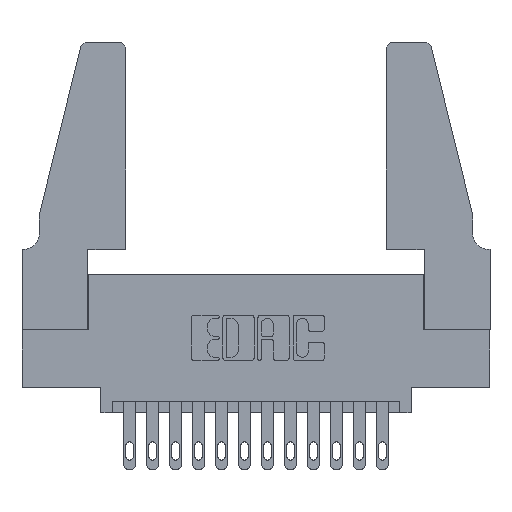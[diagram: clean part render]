
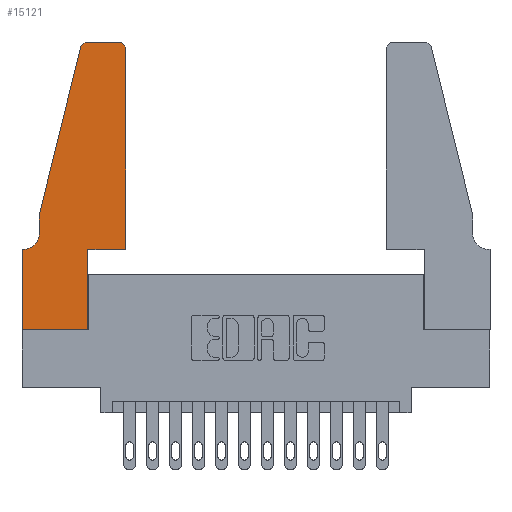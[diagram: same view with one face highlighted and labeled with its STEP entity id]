
A CAD part, top view. The second image highlights one B-rep face of the part: STEP entity #15121.
In plain terms, the highlighted planar face has unit normal (0, 0, 1).
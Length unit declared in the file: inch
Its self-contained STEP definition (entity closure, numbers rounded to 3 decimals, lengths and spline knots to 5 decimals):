
#67 = EDGE_CURVE ( 'NONE', #5300, #13426, #7095, .T. ) ;
#157 = VECTOR ( 'NONE', #8464, 39.37008 ) ;
#318 = LINE ( 'NONE', #5519, #14913 ) ;
#465 = CARTESIAN_POINT ( 'NONE',  ( 0., 0.35, 0.37 ) ) ;
#573 = EDGE_CURVE ( 'NONE', #2200, #4319, #5377, .T. ) ;
#613 = AXIS2_PLACEMENT_3D ( 'NONE', #645, #13891, #11361 ) ;
#630 = VERTEX_POINT ( 'NONE', #9015 ) ;
#645 = CARTESIAN_POINT ( 'NONE',  ( 0.284, 1.22, 0.37 ) ) ;
#835 = ORIENTED_EDGE ( 'NONE', *, *, #67, .T. ) ;
#865 = FACE_OUTER_BOUND ( 'NONE', #1805, .T. ) ;
#1190 = LINE ( 'NONE', #7786, #9736 ) ;
#1316 = EDGE_CURVE ( 'NONE', #12863, #2200, #9696, .T. ) ;
#1805 = EDGE_LOOP ( 'NONE', ( #11169, #7963, #5261, #4058, #13999, #9672, #11109, #8523, #835, #10504, #7614, #3324 ) ) ;
#1875 = DIRECTION ( 'NONE',  ( 0., -1., 0. ) ) ;
#1918 = EDGE_CURVE ( 'NONE', #13426, #11104, #13650, .T. ) ;
#2200 = VERTEX_POINT ( 'NONE', #2621 ) ;
#2281 = VECTOR ( 'NONE', #5505, 39.37008 ) ;
#2303 = EDGE_CURVE ( 'NONE', #630, #12023, #2631, .T. ) ;
#2348 = DIRECTION ( 'NONE',  ( 1., 0., 0. ) ) ;
#2621 = CARTESIAN_POINT ( 'NONE',  ( 0.284, 1.25, 0.37 ) ) ;
#2626 = AXIS2_PLACEMENT_3D ( 'NONE', #8407, #15666, #2348 ) ;
#2631 = CIRCLE ( 'NONE', #3877, 0.07 ) ;
#2777 = VECTOR ( 'NONE', #5715, 39.37008 ) ;
#3317 = DIRECTION ( 'NONE',  ( 0., 0., -1. ) ) ;
#3324 = ORIENTED_EDGE ( 'NONE', *, *, #9983, .T. ) ;
#3445 = EDGE_CURVE ( 'NONE', #5914, #4510, #318, .T. ) ;
#3466 = VECTOR ( 'NONE', #14533, 39.37008 ) ;
#3470 = EDGE_CURVE ( 'NONE', #13828, #630, #10181, .T. ) ;
#3681 = CARTESIAN_POINT ( 'NONE',  ( 0.0755, 0.35, 0.37 ) ) ;
#3877 = AXIS2_PLACEMENT_3D ( 'NONE', #9301, #3317, #5675 ) ;
#3904 = CARTESIAN_POINT ( 'NONE',  ( 0.4205, 1.25, 0.37 ) ) ;
#4052 = LINE ( 'NONE', #4678, #10135 ) ;
#4058 = ORIENTED_EDGE ( 'NONE', *, *, #3470, .T. ) ;
#4319 = VERTEX_POINT ( 'NONE', #11780 ) ;
#4510 = VERTEX_POINT ( 'NONE', #10077 ) ;
#4678 = CARTESIAN_POINT ( 'NONE',  ( 0., 0., 0.37 ) ) ;
#4879 = PLANE ( 'NONE',  #13546 ) ;
#5085 = DIRECTION ( 'NONE',  ( 1., 0., 0. ) ) ;
#5261 = ORIENTED_EDGE ( 'NONE', *, *, #14078, .T. ) ;
#5300 = VERTEX_POINT ( 'NONE', #12342 ) ;
#5377 = CIRCLE ( 'NONE', #613, 0.03 ) ;
#5505 = DIRECTION ( 'NONE',  ( -1., 0., 0. ) ) ;
#5519 = CARTESIAN_POINT ( 'NONE',  ( 0., 0., 0.37 ) ) ;
#5675 = DIRECTION ( 'NONE',  ( -1., 0., 0. ) ) ;
#5715 = DIRECTION ( 'NONE',  ( -0.239, -0.971, 0. ) ) ;
#5914 = VERTEX_POINT ( 'NONE', #465 ) ;
#6298 = CARTESIAN_POINT ( 'NONE',  ( 0., 0.35, 0.37 ) ) ;
#6673 = EDGE_CURVE ( 'NONE', #11104, #7295, #1190, .T. ) ;
#7095 = LINE ( 'NONE', #8273, #3466 ) ;
#7295 = VERTEX_POINT ( 'NONE', #11320 ) ;
#7614 = ORIENTED_EDGE ( 'NONE', *, *, #6673, .T. ) ;
#7770 = CARTESIAN_POINT ( 'NONE',  ( 0.0755, 0.5, 0.37 ) ) ;
#7786 = CARTESIAN_POINT ( 'NONE',  ( 0.4505, 0.35, 0.37 ) ) ;
#7926 = LINE ( 'NONE', #3681, #157 ) ;
#7963 = ORIENTED_EDGE ( 'NONE', *, *, #573, .T. ) ;
#7982 = CARTESIAN_POINT ( 'NONE',  ( 0.0755, 0.5, 0.37 ) ) ;
#8248 = DIRECTION ( 'NONE',  ( 1., 0., 0. ) ) ;
#8273 = CARTESIAN_POINT ( 'NONE',  ( 0.2865, 0.35, 0.37 ) ) ;
#8407 = CARTESIAN_POINT ( 'NONE',  ( 0.4205, 1.22, 0.37 ) ) ;
#8439 = DIRECTION ( 'NONE',  ( 0., 0., 1. ) ) ;
#8464 = DIRECTION ( 'NONE',  ( -1., 0., 0. ) ) ;
#8523 = ORIENTED_EDGE ( 'NONE', *, *, #10004, .T. ) ;
#8655 = CARTESIAN_POINT ( 'NONE',  ( 0.2605, 1.25, 0.37 ) ) ;
#9015 = CARTESIAN_POINT ( 'NONE',  ( 0.0755, 0.42, 0.37 ) ) ;
#9301 = CARTESIAN_POINT ( 'NONE',  ( 0.0055, 0.42, 0.37 ) ) ;
#9672 = ORIENTED_EDGE ( 'NONE', *, *, #13618, .T. ) ;
#9696 = LINE ( 'NONE', #8655, #2281 ) ;
#9736 = VECTOR ( 'NONE', #12661, 39.37008 ) ;
#9780 = CARTESIAN_POINT ( 'NONE',  ( 0.0055, 0.35, 0.37 ) ) ;
#9983 = EDGE_CURVE ( 'NONE', #7295, #12863, #10519, .T. ) ;
#10004 = EDGE_CURVE ( 'NONE', #4510, #5300, #4052, .T. ) ;
#10077 = CARTESIAN_POINT ( 'NONE',  ( 0., 0., 0.37 ) ) ;
#10135 = VECTOR ( 'NONE', #8248, 39.37008 ) ;
#10181 = LINE ( 'NONE', #14067, #11322 ) ;
#10400 = CARTESIAN_POINT ( 'NONE',  ( 0.4505, 0.35, 0.37 ) ) ;
#10504 = ORIENTED_EDGE ( 'NONE', *, *, #1918, .T. ) ;
#10519 = CIRCLE ( 'NONE', #2626, 0.03 ) ;
#10545 = CARTESIAN_POINT ( 'NONE',  ( 0.2865, 0.35, 0.37 ) ) ;
#10730 = DIRECTION ( 'NONE',  ( 0., -1., 0. ) ) ;
#11104 = VERTEX_POINT ( 'NONE', #10400 ) ;
#11109 = ORIENTED_EDGE ( 'NONE', *, *, #3445, .T. ) ;
#11169 = ORIENTED_EDGE ( 'NONE', *, *, #1316, .T. ) ;
#11320 = CARTESIAN_POINT ( 'NONE',  ( 0.4505, 1.22, 0.37 ) ) ;
#11322 = VECTOR ( 'NONE', #10730, 39.37008 ) ;
#11361 = DIRECTION ( 'NONE',  ( 1., 0., 0. ) ) ;
#11780 = CARTESIAN_POINT ( 'NONE',  ( 0.25487, 1.22718, 0.37 ) ) ;
#11892 = CARTESIAN_POINT ( 'NONE',  ( 0.4505, 0.35, 0.37 ) ) ;
#12023 = VERTEX_POINT ( 'NONE', #9780 ) ;
#12342 = CARTESIAN_POINT ( 'NONE',  ( 0.2865, 0., 0.37 ) ) ;
#12661 = DIRECTION ( 'NONE',  ( 0., 1., 0. ) ) ;
#12863 = VERTEX_POINT ( 'NONE', #3904 ) ;
#13362 = DIRECTION ( 'NONE',  ( 1., 0., 0. ) ) ;
#13426 = VERTEX_POINT ( 'NONE', #10545 ) ;
#13546 = AXIS2_PLACEMENT_3D ( 'NONE', #6298, #8439, #5085 ) ;
#13618 = EDGE_CURVE ( 'NONE', #12023, #5914, #7926, .T. ) ;
#13650 = LINE ( 'NONE', #11892, #14216 ) ;
#13828 = VERTEX_POINT ( 'NONE', #7770 ) ;
#13891 = DIRECTION ( 'NONE',  ( 0., 0., 1. ) ) ;
#13999 = ORIENTED_EDGE ( 'NONE', *, *, #2303, .T. ) ;
#14067 = CARTESIAN_POINT ( 'NONE',  ( 0.0755, 0.5, 0.37 ) ) ;
#14078 = EDGE_CURVE ( 'NONE', #4319, #13828, #14922, .T. ) ;
#14216 = VECTOR ( 'NONE', #13362, 39.37008 ) ;
#14533 = DIRECTION ( 'NONE',  ( 0., 1., 0. ) ) ;
#14913 = VECTOR ( 'NONE', #1875, 39.37008 ) ;
#14922 = LINE ( 'NONE', #7982, #2777 ) ;
#15121 = ADVANCED_FACE ( 'NONE', ( #865 ), #4879, .T. ) ;
#15666 = DIRECTION ( 'NONE',  ( 0., 0., 1. ) ) ;
